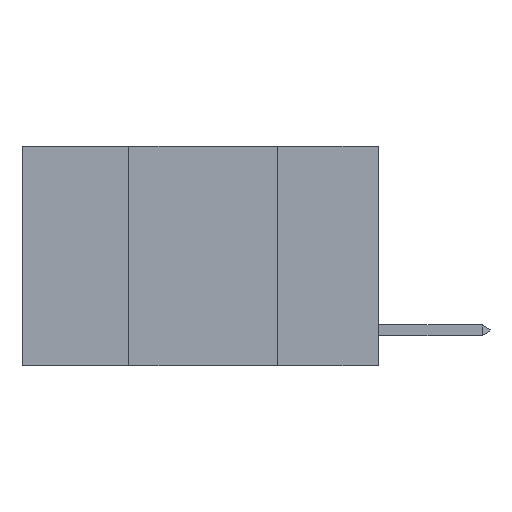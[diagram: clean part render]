
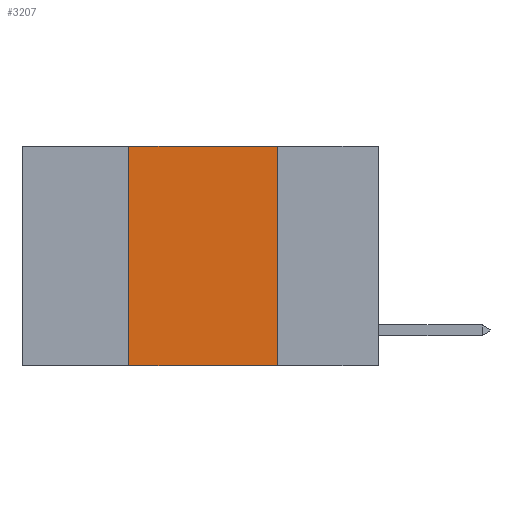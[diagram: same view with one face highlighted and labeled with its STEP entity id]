
A CAD part, left-side view. The second image highlights one B-rep face of the part: STEP entity #3207.
In plain terms, the highlighted planar face has unit normal (-1, 0, 0).
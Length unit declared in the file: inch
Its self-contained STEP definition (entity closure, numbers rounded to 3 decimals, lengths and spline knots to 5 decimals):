
#224 = ORIENTED_EDGE ( 'NONE', *, *, #6927, .F. ) ;
#651 = FACE_OUTER_BOUND ( 'NONE', #11454, .T. ) ;
#1697 = CARTESIAN_POINT ( 'NONE',  ( 0., 0.17, -0.37 ) ) ;
#2280 = VERTEX_POINT ( 'NONE', #3390 ) ;
#3207 = ADVANCED_FACE ( 'NONE', ( #651 ), #13207, .F. ) ;
#3390 = CARTESIAN_POINT ( 'NONE',  ( 0., 0.42, -0.37 ) ) ;
#3837 = LINE ( 'NONE', #9655, #12672 ) ;
#4535 = DIRECTION ( 'NONE',  ( 0., 0., 1. ) ) ;
#4778 = CARTESIAN_POINT ( 'NONE',  ( 0., 0.17, 0. ) ) ;
#6248 = CARTESIAN_POINT ( 'NONE',  ( 0., 0.42, 0. ) ) ;
#6827 = CARTESIAN_POINT ( 'NONE',  ( 0., 0.6, -0.37 ) ) ;
#6927 = EDGE_CURVE ( 'NONE', #2280, #11316, #7488, .T. ) ;
#7299 = LINE ( 'NONE', #16297, #16937 ) ;
#7488 = LINE ( 'NONE', #6248, #10983 ) ;
#8526 = LINE ( 'NONE', #6827, #13566 ) ;
#9655 = CARTESIAN_POINT ( 'NONE',  ( 0., 0.17, 0. ) ) ;
#10398 = CARTESIAN_POINT ( 'NONE',  ( 0., 0.6, 0. ) ) ;
#10952 = EDGE_CURVE ( 'NONE', #11316, #13763, #7299, .T. ) ;
#10983 = VECTOR ( 'NONE', #4535, 39.37008 ) ;
#11198 = EDGE_CURVE ( 'NONE', #2280, #11778, #8526, .T. ) ;
#11316 = VERTEX_POINT ( 'NONE', #13215 ) ;
#11454 = EDGE_LOOP ( 'NONE', ( #16737, #16143, #224, #15882 ) ) ;
#11778 = VERTEX_POINT ( 'NONE', #1697 ) ;
#12437 = DIRECTION ( 'NONE',  ( 1., 0., 0. ) ) ;
#12672 = VECTOR ( 'NONE', #15319, 39.37008 ) ;
#13207 = PLANE ( 'NONE',  #18130 ) ;
#13215 = CARTESIAN_POINT ( 'NONE',  ( 0., 0.42, 0. ) ) ;
#13566 = VECTOR ( 'NONE', #16958, 39.37008 ) ;
#13763 = VERTEX_POINT ( 'NONE', #4778 ) ;
#15161 = EDGE_CURVE ( 'NONE', #13763, #11778, #3837, .T. ) ;
#15319 = DIRECTION ( 'NONE',  ( 0., 0., -1. ) ) ;
#15882 = ORIENTED_EDGE ( 'NONE', *, *, #11198, .T. ) ;
#16143 = ORIENTED_EDGE ( 'NONE', *, *, #10952, .F. ) ;
#16202 = DIRECTION ( 'NONE',  ( 0., -1., 0. ) ) ;
#16297 = CARTESIAN_POINT ( 'NONE',  ( 0., 0.6, 0. ) ) ;
#16737 = ORIENTED_EDGE ( 'NONE', *, *, #15161, .F. ) ;
#16937 = VECTOR ( 'NONE', #16202, 39.37008 ) ;
#16958 = DIRECTION ( 'NONE',  ( 0., -1., 0. ) ) ;
#18130 = AXIS2_PLACEMENT_3D ( 'NONE', #10398, #12437, #18207 ) ;
#18207 = DIRECTION ( 'NONE',  ( 0., 0., -1. ) ) ;
